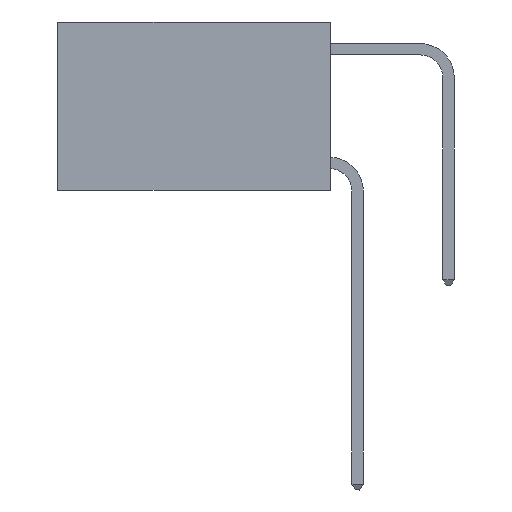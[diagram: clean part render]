
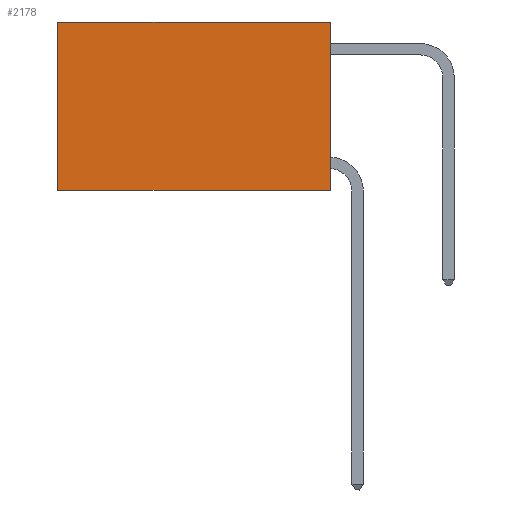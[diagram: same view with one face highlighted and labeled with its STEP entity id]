
A CAD part, left-side view. The second image highlights one B-rep face of the part: STEP entity #2178.
In plain terms, the highlighted planar face has unit normal (-1, 0, 0).
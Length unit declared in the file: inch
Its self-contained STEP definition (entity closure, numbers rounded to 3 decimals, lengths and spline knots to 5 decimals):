
#979 = AXIS2_PLACEMENT_3D ( 'NONE', #1746, #9406, #7970 ) ;
#1400 = DIRECTION ( 'NONE',  ( 0., 1., 0. ) ) ;
#1614 = DIRECTION ( 'NONE',  ( 0., 0., -1. ) ) ;
#1746 = CARTESIAN_POINT ( 'NONE',  ( 0.2625, 0., 0. ) ) ;
#2178 = ADVANCED_FACE ( 'NONE', ( #11125 ), #7101, .F. ) ;
#2459 = VERTEX_POINT ( 'NONE', #3178 ) ;
#3178 = CARTESIAN_POINT ( 'NONE',  ( 0.2625, 0.6, 0. ) ) ;
#3999 = ORIENTED_EDGE ( 'NONE', *, *, #9921, .T. ) ;
#4242 = ORIENTED_EDGE ( 'NONE', *, *, #8428, .F. ) ;
#4660 = ORIENTED_EDGE ( 'NONE', *, *, #6646, .F. ) ;
#4717 = ORIENTED_EDGE ( 'NONE', *, *, #7920, .T. ) ;
#6152 = LINE ( 'NONE', #11720, #8432 ) ;
#6186 = EDGE_LOOP ( 'NONE', ( #3999, #4242, #4660, #4717 ) ) ;
#6227 = CARTESIAN_POINT ( 'NONE',  ( 0.2625, 0.6, -0.37 ) ) ;
#6322 = VECTOR ( 'NONE', #1614, 39.37008 ) ;
#6646 = EDGE_CURVE ( 'NONE', #8502, #9153, #11549, .T. ) ;
#6799 = DIRECTION ( 'NONE',  ( 0., 1., 0. ) ) ;
#7101 = PLANE ( 'NONE',  #979 ) ;
#7493 = CARTESIAN_POINT ( 'NONE',  ( 0.2625, 0., 0. ) ) ;
#7521 = CARTESIAN_POINT ( 'NONE',  ( 0.2625, 0., -0.37 ) ) ;
#7563 = CARTESIAN_POINT ( 'NONE',  ( 0.2625, 0., 0. ) ) ;
#7920 = EDGE_CURVE ( 'NONE', #8502, #2459, #6152, .T. ) ;
#7970 = DIRECTION ( 'NONE',  ( 0., 0., -1. ) ) ;
#8428 = EDGE_CURVE ( 'NONE', #9153, #10042, #12457, .T. ) ;
#8432 = VECTOR ( 'NONE', #6799, 39.37008 ) ;
#8502 = VERTEX_POINT ( 'NONE', #7493 ) ;
#9004 = VECTOR ( 'NONE', #10810, 39.37008 ) ;
#9153 = VERTEX_POINT ( 'NONE', #7521 ) ;
#9406 = DIRECTION ( 'NONE',  ( 1., 0., 0. ) ) ;
#9502 = VECTOR ( 'NONE', #1400, 39.37008 ) ;
#9738 = CARTESIAN_POINT ( 'NONE',  ( 0.2625, 0.6, 0. ) ) ;
#9921 = EDGE_CURVE ( 'NONE', #2459, #10042, #11629, .T. ) ;
#10042 = VERTEX_POINT ( 'NONE', #6227 ) ;
#10810 = DIRECTION ( 'NONE',  ( 0., 0., -1. ) ) ;
#11125 = FACE_OUTER_BOUND ( 'NONE', #6186, .T. ) ;
#11549 = LINE ( 'NONE', #7563, #6322 ) ;
#11629 = LINE ( 'NONE', #9738, #9004 ) ;
#11720 = CARTESIAN_POINT ( 'NONE',  ( 0.2625, 0., 0. ) ) ;
#12420 = CARTESIAN_POINT ( 'NONE',  ( 0.2625, 0., -0.37 ) ) ;
#12457 = LINE ( 'NONE', #12420, #9502 ) ;
